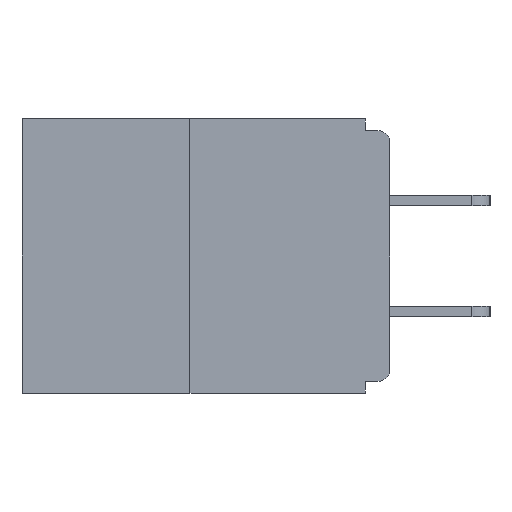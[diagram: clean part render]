
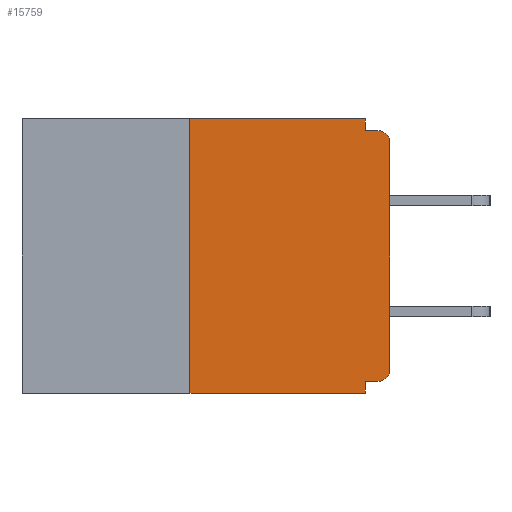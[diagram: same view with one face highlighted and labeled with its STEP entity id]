
A CAD part, left-side view. The second image highlights one B-rep face of the part: STEP entity #15759.
In plain terms, the highlighted planar face has unit normal (-1, 0, 0).
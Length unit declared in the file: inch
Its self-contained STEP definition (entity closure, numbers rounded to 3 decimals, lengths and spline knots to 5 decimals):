
#143 = VERTEX_POINT ( 'NONE', #8096 ) ;
#648 = CARTESIAN_POINT ( 'NONE',  ( 0., 0., -0.015 ) ) ;
#760 = LINE ( 'NONE', #9267, #11385 ) ;
#1269 = EDGE_CURVE ( 'NONE', #25904, #4851, #760, .T. ) ;
#1650 = VECTOR ( 'NONE', #24029, 39.37008 ) ;
#1765 = EDGE_CURVE ( 'NONE', #143, #9901, #6416, .T. ) ;
#1941 = LINE ( 'NONE', #4311, #14868 ) ;
#2082 = ORIENTED_EDGE ( 'NONE', *, *, #1269, .F. ) ;
#2141 = ORIENTED_EDGE ( 'NONE', *, *, #16473, .F. ) ;
#2318 = LINE ( 'NONE', #648, #19680 ) ;
#2991 = DIRECTION ( 'NONE',  ( 1., 0., 0. ) ) ;
#3336 = VECTOR ( 'NONE', #24422, 39.37008 ) ;
#3666 = CARTESIAN_POINT ( 'NONE',  ( 0., 0.46, -0.343 ) ) ;
#3931 = DIRECTION ( 'NONE',  ( 0., 0., 1. ) ) ;
#4184 = DIRECTION ( 'NONE',  ( 0., 0., 1. ) ) ;
#4311 = CARTESIAN_POINT ( 'NONE',  ( 0., 0.031, 0. ) ) ;
#4784 = ORIENTED_EDGE ( 'NONE', *, *, #22192, .T. ) ;
#4831 = DIRECTION ( 'NONE',  ( 0., -1., 0. ) ) ;
#4851 = VERTEX_POINT ( 'NONE', #24387 ) ;
#5925 = VECTOR ( 'NONE', #4184, 39.37008 ) ;
#6040 = DIRECTION ( 'NONE',  ( -1., 0., 0. ) ) ;
#6260 = AXIS2_PLACEMENT_3D ( 'NONE', #9141, #2991, #23873 ) ;
#6278 = EDGE_LOOP ( 'NONE', ( #2082, #8011, #9898, #17321, #23302, #13471, #4784, #15755, #18116, #2141 ) ) ;
#6416 = CIRCLE ( 'NONE', #20217, 0.015 ) ;
#6423 = LINE ( 'NONE', #18600, #5925 ) ;
#7181 = DIRECTION ( 'NONE',  ( 0., -1., 0. ) ) ;
#7847 = CARTESIAN_POINT ( 'NONE',  ( 0., 0., 0. ) ) ;
#8011 = ORIENTED_EDGE ( 'NONE', *, *, #14513, .F. ) ;
#8096 = CARTESIAN_POINT ( 'NONE',  ( 0., 0., -0.03 ) ) ;
#9141 = CARTESIAN_POINT ( 'NONE',  ( 0., 0.46, 0. ) ) ;
#9267 = CARTESIAN_POINT ( 'NONE',  ( 0., 0.46, 0. ) ) ;
#9782 = VERTEX_POINT ( 'NONE', #22176 ) ;
#9898 = ORIENTED_EDGE ( 'NONE', *, *, #21943, .T. ) ;
#9901 = VERTEX_POINT ( 'NONE', #10059 ) ;
#10059 = CARTESIAN_POINT ( 'NONE',  ( 0., 0.015, -0.015 ) ) ;
#10854 = CARTESIAN_POINT ( 'NONE',  ( 0., 0.031, -0.343 ) ) ;
#11115 = FACE_OUTER_BOUND ( 'NONE', #6278, .T. ) ;
#11385 = VECTOR ( 'NONE', #7181, 39.37008 ) ;
#11562 = CARTESIAN_POINT ( 'NONE',  ( 0., 0.25, 0. ) ) ;
#11726 = CARTESIAN_POINT ( 'NONE',  ( 0., 0., -0.328 ) ) ;
#12082 = CARTESIAN_POINT ( 'NONE',  ( 0., 0.015, -0.313 ) ) ;
#12325 = DIRECTION ( 'NONE',  ( 0., 0., -1. ) ) ;
#13471 = ORIENTED_EDGE ( 'NONE', *, *, #26603, .T. ) ;
#14304 = VERTEX_POINT ( 'NONE', #16112 ) ;
#14513 = EDGE_CURVE ( 'NONE', #24944, #25904, #6423, .T. ) ;
#14598 = DIRECTION ( 'NONE',  ( 0., 0., -1. ) ) ;
#14832 = EDGE_CURVE ( 'NONE', #19662, #23040, #16211, .T. ) ;
#14868 = VECTOR ( 'NONE', #12325, 39.37008 ) ;
#15608 = LINE ( 'NONE', #10854, #1650 ) ;
#15755 = ORIENTED_EDGE ( 'NONE', *, *, #1765, .T. ) ;
#15759 = ADVANCED_FACE ( 'NONE', ( #11115 ), #26383, .F. ) ;
#16110 = CARTESIAN_POINT ( 'NONE',  ( 0., 0.25, -0.343 ) ) ;
#16112 = CARTESIAN_POINT ( 'NONE',  ( 0., 0., -0.313 ) ) ;
#16191 = DIRECTION ( 'NONE',  ( 0., 0., -1. ) ) ;
#16211 = LINE ( 'NONE', #11726, #27008 ) ;
#16473 = EDGE_CURVE ( 'NONE', #4851, #25877, #1941, .T. ) ;
#16828 = CARTESIAN_POINT ( 'NONE',  ( 0., 0.015, -0.328 ) ) ;
#17011 = EDGE_CURVE ( 'NONE', #25877, #9901, #2318, .T. ) ;
#17189 = VECTOR ( 'NONE', #3931, 39.37008 ) ;
#17321 = ORIENTED_EDGE ( 'NONE', *, *, #27166, .F. ) ;
#17559 = CARTESIAN_POINT ( 'NONE',  ( 0., 0.031, -0.328 ) ) ;
#18116 = ORIENTED_EDGE ( 'NONE', *, *, #17011, .F. ) ;
#18600 = CARTESIAN_POINT ( 'NONE',  ( 0., 0.25, 0. ) ) ;
#18981 = CIRCLE ( 'NONE', #19433, 0.015 ) ;
#19433 = AXIS2_PLACEMENT_3D ( 'NONE', #12082, #6040, #14598 ) ;
#19662 = VERTEX_POINT ( 'NONE', #16828 ) ;
#19680 = VECTOR ( 'NONE', #4831, 39.37008 ) ;
#20217 = AXIS2_PLACEMENT_3D ( 'NONE', #22398, #26987, #16191 ) ;
#21943 = EDGE_CURVE ( 'NONE', #24944, #9782, #22758, .T. ) ;
#22176 = CARTESIAN_POINT ( 'NONE',  ( 0., 0.031, -0.343 ) ) ;
#22192 = EDGE_CURVE ( 'NONE', #14304, #143, #24819, .T. ) ;
#22398 = CARTESIAN_POINT ( 'NONE',  ( 0., 0.015, -0.03 ) ) ;
#22758 = LINE ( 'NONE', #3666, #3336 ) ;
#23040 = VERTEX_POINT ( 'NONE', #17559 ) ;
#23302 = ORIENTED_EDGE ( 'NONE', *, *, #14832, .F. ) ;
#23873 = DIRECTION ( 'NONE',  ( 0., 0., -1. ) ) ;
#23905 = CARTESIAN_POINT ( 'NONE',  ( 0., 0.031, -0.015 ) ) ;
#24029 = DIRECTION ( 'NONE',  ( 0., 0., -1. ) ) ;
#24387 = CARTESIAN_POINT ( 'NONE',  ( 0., 0.031, 0. ) ) ;
#24422 = DIRECTION ( 'NONE',  ( 0., -1., 0. ) ) ;
#24819 = LINE ( 'NONE', #7847, #17189 ) ;
#24944 = VERTEX_POINT ( 'NONE', #16110 ) ;
#25877 = VERTEX_POINT ( 'NONE', #23905 ) ;
#25904 = VERTEX_POINT ( 'NONE', #11562 ) ;
#26314 = DIRECTION ( 'NONE',  ( 0., 1., 0. ) ) ;
#26383 = PLANE ( 'NONE',  #6260 ) ;
#26603 = EDGE_CURVE ( 'NONE', #19662, #14304, #18981, .T. ) ;
#26987 = DIRECTION ( 'NONE',  ( -1., 0., 0. ) ) ;
#27008 = VECTOR ( 'NONE', #26314, 39.37008 ) ;
#27166 = EDGE_CURVE ( 'NONE', #23040, #9782, #15608, .T. ) ;
